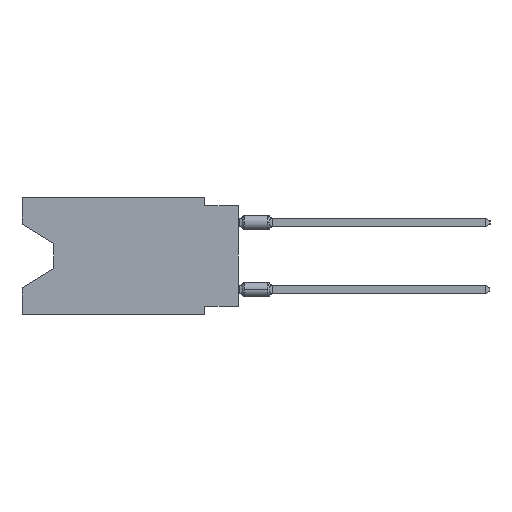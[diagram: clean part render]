
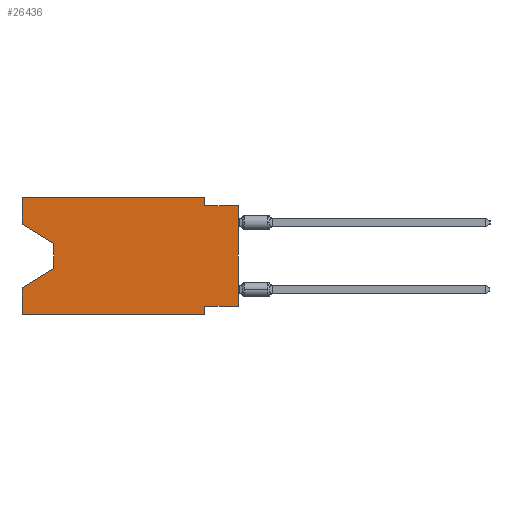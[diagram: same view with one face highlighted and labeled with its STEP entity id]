
A CAD part, left-side view. The second image highlights one B-rep face of the part: STEP entity #26436.
In plain terms, the highlighted planar face has unit normal (-1, 0, 0).
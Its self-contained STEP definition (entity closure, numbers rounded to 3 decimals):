
#325 = VECTOR ( 'NONE', #42731, 1000. ) ;
#739 = VECTOR ( 'NONE', #18301, 1000. ) ;
#772 = CARTESIAN_POINT ( 'NONE',  ( 0., 2.54, -8.255 ) ) ;
#1803 = CARTESIAN_POINT ( 'NONE',  ( 0., 16.383, -2.038 ) ) ;
#1963 = ORIENTED_EDGE ( 'NONE', *, *, #68249, .F. ) ;
#2410 = EDGE_CURVE ( 'NONE', #49224, #22419, #15170, .T. ) ;
#3194 = LINE ( 'NONE', #8411, #26164 ) ;
#3312 = CARTESIAN_POINT ( 'NONE',  ( 0., 0., -8.255 ) ) ;
#3623 = CARTESIAN_POINT ( 'NONE',  ( 0., 16.383, 0. ) ) ;
#4562 = LINE ( 'NONE', #45724, #62099 ) ;
#4772 = VECTOR ( 'NONE', #61825, 1000. ) ;
#7780 = LINE ( 'NONE', #23479, #4772 ) ;
#8203 = CARTESIAN_POINT ( 'NONE',  ( 0., 16.383, -8.89 ) ) ;
#8411 = CARTESIAN_POINT ( 'NONE',  ( 0., 16.383, 0. ) ) ;
#9521 = DIRECTION ( 'NONE',  ( 0., 0., -1. ) ) ;
#9745 = CARTESIAN_POINT ( 'NONE',  ( 0., 16.383, -8.89 ) ) ;
#10292 = EDGE_LOOP ( 'NONE', ( #35539, #61666, #15641, #18971, #22804, #25271, #12751, #11599, #42322, #31823, #19957, #1963 ) ) ;
#10823 = VECTOR ( 'NONE', #49042, 1000. ) ;
#11599 = ORIENTED_EDGE ( 'NONE', *, *, #17950, .T. ) ;
#12105 = VERTEX_POINT ( 'NONE', #19284 ) ;
#12361 = LINE ( 'NONE', #55291, #33577 ) ;
#12751 = ORIENTED_EDGE ( 'NONE', *, *, #63171, .F. ) ;
#12991 = VECTOR ( 'NONE', #9521, 1000. ) ;
#13087 = VERTEX_POINT ( 'NONE', #63644 ) ;
#13312 = DIRECTION ( 'NONE',  ( 0., 0.855, -0.519 ) ) ;
#13786 = EDGE_CURVE ( 'NONE', #61459, #29192, #3194, .T. ) ;
#15170 = LINE ( 'NONE', #31242, #325 ) ;
#15641 = ORIENTED_EDGE ( 'NONE', *, *, #46295, .T. ) ;
#16717 = VECTOR ( 'NONE', #51396, 1000. ) ;
#17470 = DIRECTION ( 'NONE',  ( 0., 0., 1. ) ) ;
#17950 = EDGE_CURVE ( 'NONE', #38819, #31246, #55489, .T. ) ;
#18301 = DIRECTION ( 'NONE',  ( 0., 1., 0. ) ) ;
#18971 = ORIENTED_EDGE ( 'NONE', *, *, #13786, .F. ) ;
#19284 = CARTESIAN_POINT ( 'NONE',  ( 0., 16.383, 0. ) ) ;
#19957 = ORIENTED_EDGE ( 'NONE', *, *, #64310, .F. ) ;
#19996 = LINE ( 'NONE', #56633, #12991 ) ;
#22419 = VERTEX_POINT ( 'NONE', #38060 ) ;
#22621 = PLANE ( 'NONE',  #37733 ) ;
#22804 = ORIENTED_EDGE ( 'NONE', *, *, #36007, .T. ) ;
#23479 = CARTESIAN_POINT ( 'NONE',  ( 0., 16.383, -2.038 ) ) ;
#25271 = ORIENTED_EDGE ( 'NONE', *, *, #2410, .F. ) ;
#26164 = VECTOR ( 'NONE', #65622, 1000. ) ;
#26436 = ADVANCED_FACE ( 'NONE', ( #49492 ), #22621, .F. ) ;
#27528 = CARTESIAN_POINT ( 'NONE',  ( 0., 16.383, 0. ) ) ;
#29192 = VERTEX_POINT ( 'NONE', #31902 ) ;
#31242 = CARTESIAN_POINT ( 'NONE',  ( 0., 2.54, -8.89 ) ) ;
#31246 = VERTEX_POINT ( 'NONE', #61073 ) ;
#31823 = ORIENTED_EDGE ( 'NONE', *, *, #35522, .F. ) ;
#31902 = CARTESIAN_POINT ( 'NONE',  ( 0., 16.383, -6.852 ) ) ;
#33577 = VECTOR ( 'NONE', #33654, 1000. ) ;
#33654 = DIRECTION ( 'NONE',  ( 0., 0., -1. ) ) ;
#34004 = VERTEX_POINT ( 'NONE', #1803 ) ;
#35522 = EDGE_CURVE ( 'NONE', #13087, #47347, #19996, .T. ) ;
#35539 = ORIENTED_EDGE ( 'NONE', *, *, #48967, .T. ) ;
#36007 = EDGE_CURVE ( 'NONE', #61459, #22419, #55986, .T. ) ;
#37733 = AXIS2_PLACEMENT_3D ( 'NONE', #27528, #44246, #59262 ) ;
#38060 = CARTESIAN_POINT ( 'NONE',  ( 0., 2.54, -8.89 ) ) ;
#38819 = VERTEX_POINT ( 'NONE', #49301 ) ;
#39224 = LINE ( 'NONE', #3312, #739 ) ;
#39427 = CARTESIAN_POINT ( 'NONE',  ( 0., 0., 0. ) ) ;
#39643 = LINE ( 'NONE', #60919, #67465 ) ;
#40875 = EDGE_CURVE ( 'NONE', #47347, #31246, #39643, .T. ) ;
#42322 = ORIENTED_EDGE ( 'NONE', *, *, #40875, .F. ) ;
#42731 = DIRECTION ( 'NONE',  ( 0., 0., -1. ) ) ;
#44246 = DIRECTION ( 'NONE',  ( 1., 0., 0. ) ) ;
#44525 = DIRECTION ( 'NONE',  ( 0., -1., 0. ) ) ;
#44779 = LINE ( 'NONE', #3623, #16717 ) ;
#45724 = CARTESIAN_POINT ( 'NONE',  ( 0., 16.383, 0. ) ) ;
#46295 = EDGE_CURVE ( 'NONE', #46989, #29192, #62141, .T. ) ;
#46545 = VERTEX_POINT ( 'NONE', #54412 ) ;
#46989 = VERTEX_POINT ( 'NONE', #60247 ) ;
#47347 = VERTEX_POINT ( 'NONE', #54249 ) ;
#47569 = EDGE_CURVE ( 'NONE', #46545, #46989, #12361, .T. ) ;
#48967 = EDGE_CURVE ( 'NONE', #34004, #46545, #7780, .T. ) ;
#49042 = DIRECTION ( 'NONE',  ( 0., -1., 0. ) ) ;
#49224 = VERTEX_POINT ( 'NONE', #772 ) ;
#49301 = CARTESIAN_POINT ( 'NONE',  ( 0., 0., -8.255 ) ) ;
#49492 = FACE_OUTER_BOUND ( 'NONE', #10292, .T. ) ;
#51396 = DIRECTION ( 'NONE',  ( 0., 0., 1. ) ) ;
#54249 = CARTESIAN_POINT ( 'NONE',  ( 0., 2.54, -0.635 ) ) ;
#54412 = CARTESIAN_POINT ( 'NONE',  ( 0., 13.97, -3.505 ) ) ;
#55291 = CARTESIAN_POINT ( 'NONE',  ( 0., 13.97, -3.505 ) ) ;
#55489 = LINE ( 'NONE', #39427, #61046 ) ;
#55986 = LINE ( 'NONE', #8203, #10823 ) ;
#56633 = CARTESIAN_POINT ( 'NONE',  ( 0., 2.54, 0. ) ) ;
#56925 = CARTESIAN_POINT ( 'NONE',  ( 0., 13.97, -5.385 ) ) ;
#59262 = DIRECTION ( 'NONE',  ( 0., 0., -1. ) ) ;
#60247 = CARTESIAN_POINT ( 'NONE',  ( 0., 13.97, -5.385 ) ) ;
#60919 = CARTESIAN_POINT ( 'NONE',  ( 0., 0., -0.635 ) ) ;
#61046 = VECTOR ( 'NONE', #17470, 1000. ) ;
#61073 = CARTESIAN_POINT ( 'NONE',  ( 0., 0., -0.635 ) ) ;
#61459 = VERTEX_POINT ( 'NONE', #9745 ) ;
#61666 = ORIENTED_EDGE ( 'NONE', *, *, #47569, .T. ) ;
#61825 = DIRECTION ( 'NONE',  ( 0., -0.855, -0.519 ) ) ;
#62099 = VECTOR ( 'NONE', #66982, 1000. ) ;
#62141 = LINE ( 'NONE', #56925, #66190 ) ;
#63171 = EDGE_CURVE ( 'NONE', #38819, #49224, #39224, .T. ) ;
#63644 = CARTESIAN_POINT ( 'NONE',  ( 0., 2.54, 0. ) ) ;
#64310 = EDGE_CURVE ( 'NONE', #12105, #13087, #4562, .T. ) ;
#65622 = DIRECTION ( 'NONE',  ( 0., 0., 1. ) ) ;
#66190 = VECTOR ( 'NONE', #13312, 1000. ) ;
#66982 = DIRECTION ( 'NONE',  ( 0., -1., 0. ) ) ;
#67465 = VECTOR ( 'NONE', #44525, 1000. ) ;
#68249 = EDGE_CURVE ( 'NONE', #34004, #12105, #44779, .T. ) ;
